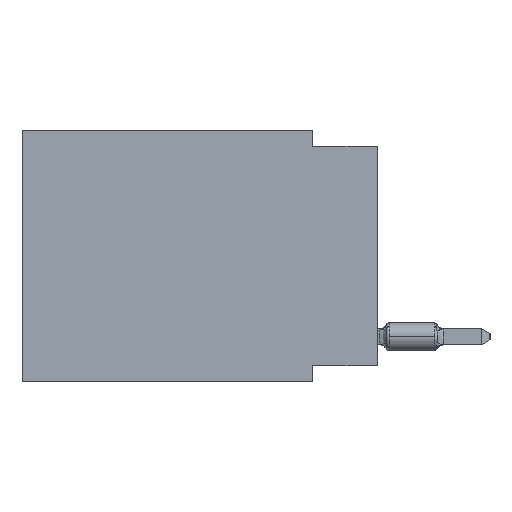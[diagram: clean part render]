
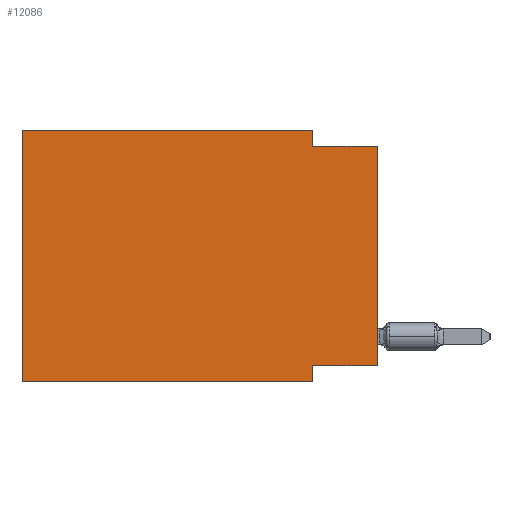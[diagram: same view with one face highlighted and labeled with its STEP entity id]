
A CAD part, left-side view. The second image highlights one B-rep face of the part: STEP entity #12086.
In plain terms, the highlighted planar face has unit normal (-1, 0, 0).
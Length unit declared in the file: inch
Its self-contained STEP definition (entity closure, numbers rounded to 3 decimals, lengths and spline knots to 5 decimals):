
#674 = FACE_OUTER_BOUND ( 'NONE', #8968, .T. ) ;
#1227 = DIRECTION ( 'NONE',  ( 0., 0., 1. ) ) ;
#1307 = CARTESIAN_POINT ( 'NONE',  ( 0., 0., -0.365 ) ) ;
#1591 = EDGE_CURVE ( 'NONE', #23410, #30502, #18101, .T. ) ;
#1804 = VERTEX_POINT ( 'NONE', #29384 ) ;
#1861 = CARTESIAN_POINT ( 'NONE',  ( 0., 0.55, 0. ) ) ;
#2399 = CARTESIAN_POINT ( 'NONE',  ( 0., 0.55, -0.39 ) ) ;
#4182 = VECTOR ( 'NONE', #12695, 39.37008 ) ;
#4187 = CARTESIAN_POINT ( 'NONE',  ( 0., 0.1, -0.39 ) ) ;
#4405 = AXIS2_PLACEMENT_3D ( 'NONE', #5630, #7957, #22207 ) ;
#4544 = VECTOR ( 'NONE', #1227, 39.37008 ) ;
#5234 = ORIENTED_EDGE ( 'NONE', *, *, #18658, .F. ) ;
#5630 = CARTESIAN_POINT ( 'NONE',  ( 0., 0.55, 0. ) ) ;
#5774 = LINE ( 'NONE', #24669, #20833 ) ;
#5888 = ORIENTED_EDGE ( 'NONE', *, *, #1591, .T. ) ;
#6724 = VERTEX_POINT ( 'NONE', #27385 ) ;
#7059 = LINE ( 'NONE', #2399, #26170 ) ;
#7957 = DIRECTION ( 'NONE',  ( 1., 0., 0. ) ) ;
#7965 = EDGE_CURVE ( 'NONE', #24205, #30502, #16388, .T. ) ;
#8062 = CARTESIAN_POINT ( 'NONE',  ( 0., 0., -0.365 ) ) ;
#8814 = CARTESIAN_POINT ( 'NONE',  ( 0., 0., 0. ) ) ;
#8968 = EDGE_LOOP ( 'NONE', ( #5888, #10466, #26878, #10249, #15626, #9813, #26502, #5234 ) ) ;
#9665 = EDGE_CURVE ( 'NONE', #6724, #22946, #26636, .T. ) ;
#9813 = ORIENTED_EDGE ( 'NONE', *, *, #11603, .T. ) ;
#9966 = VECTOR ( 'NONE', #26285, 39.37008 ) ;
#10249 = ORIENTED_EDGE ( 'NONE', *, *, #30310, .F. ) ;
#10466 = ORIENTED_EDGE ( 'NONE', *, *, #7965, .F. ) ;
#11603 = EDGE_CURVE ( 'NONE', #26642, #22946, #7059, .T. ) ;
#12086 = ADVANCED_FACE ( 'NONE', ( #674 ), #29172, .F. ) ;
#12695 = DIRECTION ( 'NONE',  ( 0., 1., 0. ) ) ;
#13582 = CARTESIAN_POINT ( 'NONE',  ( 0., 0.1, -0.025 ) ) ;
#13701 = CARTESIAN_POINT ( 'NONE',  ( 0., 0., -0.025 ) ) ;
#13728 = DIRECTION ( 'NONE',  ( 0., 0., 1. ) ) ;
#13863 = DIRECTION ( 'NONE',  ( 0., -1., 0. ) ) ;
#13908 = DIRECTION ( 'NONE',  ( 0., -1., 0. ) ) ;
#14123 = VECTOR ( 'NONE', #13908, 39.37008 ) ;
#14184 = VECTOR ( 'NONE', #27098, 39.37008 ) ;
#15525 = DIRECTION ( 'NONE',  ( 0., 0., -1. ) ) ;
#15626 = ORIENTED_EDGE ( 'NONE', *, *, #20489, .F. ) ;
#16388 = LINE ( 'NONE', #18558, #14123 ) ;
#16829 = LINE ( 'NONE', #21783, #9966 ) ;
#18101 = LINE ( 'NONE', #8814, #4544 ) ;
#18558 = CARTESIAN_POINT ( 'NONE',  ( 0., 0., -0.025 ) ) ;
#18658 = EDGE_CURVE ( 'NONE', #23410, #6724, #26969, .T. ) ;
#20489 = EDGE_CURVE ( 'NONE', #26642, #26457, #23795, .T. ) ;
#20833 = VECTOR ( 'NONE', #15525, 39.37008 ) ;
#21783 = CARTESIAN_POINT ( 'NONE',  ( 0., 0.55, 0. ) ) ;
#22207 = DIRECTION ( 'NONE',  ( 0., 0., -1. ) ) ;
#22946 = VERTEX_POINT ( 'NONE', #4187 ) ;
#23234 = CARTESIAN_POINT ( 'NONE',  ( 0., 0.55, -0.39 ) ) ;
#23410 = VERTEX_POINT ( 'NONE', #1307 ) ;
#23795 = LINE ( 'NONE', #30296, #27009 ) ;
#24205 = VERTEX_POINT ( 'NONE', #13582 ) ;
#24616 = CARTESIAN_POINT ( 'NONE',  ( 0., 0.1, -0.39 ) ) ;
#24669 = CARTESIAN_POINT ( 'NONE',  ( 0., 0.1, 0. ) ) ;
#26170 = VECTOR ( 'NONE', #13863, 39.37008 ) ;
#26285 = DIRECTION ( 'NONE',  ( 0., -1., 0. ) ) ;
#26457 = VERTEX_POINT ( 'NONE', #1861 ) ;
#26502 = ORIENTED_EDGE ( 'NONE', *, *, #9665, .F. ) ;
#26636 = LINE ( 'NONE', #24616, #14184 ) ;
#26642 = VERTEX_POINT ( 'NONE', #23234 ) ;
#26878 = ORIENTED_EDGE ( 'NONE', *, *, #27995, .F. ) ;
#26969 = LINE ( 'NONE', #8062, #4182 ) ;
#27009 = VECTOR ( 'NONE', #13728, 39.37008 ) ;
#27098 = DIRECTION ( 'NONE',  ( 0., 0., -1. ) ) ;
#27385 = CARTESIAN_POINT ( 'NONE',  ( 0., 0.1, -0.365 ) ) ;
#27995 = EDGE_CURVE ( 'NONE', #1804, #24205, #5774, .T. ) ;
#29172 = PLANE ( 'NONE',  #4405 ) ;
#29384 = CARTESIAN_POINT ( 'NONE',  ( 0., 0.1, 0. ) ) ;
#30296 = CARTESIAN_POINT ( 'NONE',  ( 0., 0.55, 0. ) ) ;
#30310 = EDGE_CURVE ( 'NONE', #26457, #1804, #16829, .T. ) ;
#30502 = VERTEX_POINT ( 'NONE', #13701 ) ;
